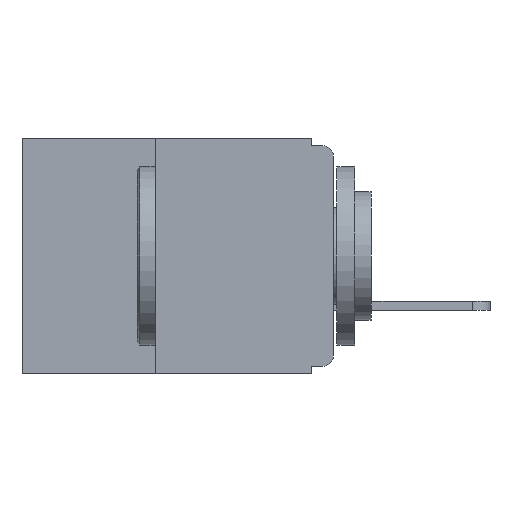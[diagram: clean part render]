
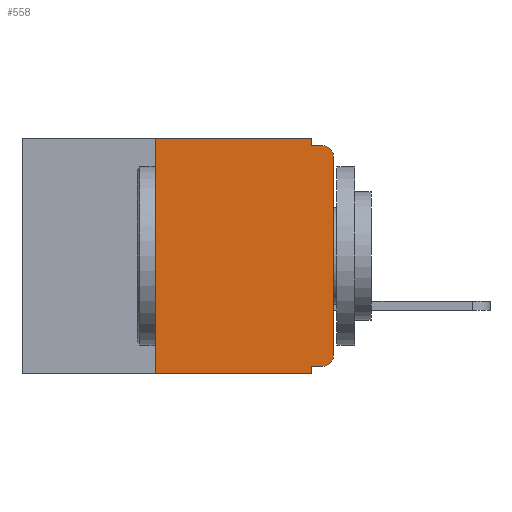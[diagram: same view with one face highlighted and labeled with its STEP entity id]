
A CAD part, left-side view. The second image highlights one B-rep face of the part: STEP entity #558.
In plain terms, the highlighted planar face has unit normal (-1, 0, 0).
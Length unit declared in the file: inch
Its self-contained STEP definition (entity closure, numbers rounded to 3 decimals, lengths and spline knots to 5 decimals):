
#59 = CARTESIAN_POINT ( 'NONE',  ( 0., 0.031, -0.01 ) ) ;
#419 = VERTEX_POINT ( 'NONE', #4689 ) ;
#448 = CARTESIAN_POINT ( 'NONE',  ( 0., 0.015, -0.025 ) ) ;
#558 = ADVANCED_FACE ( 'NONE', ( #9040 ), #2734, .F. ) ;
#847 = EDGE_LOOP ( 'NONE', ( #12731, #2607, #6334, #4284, #2708, #13436, #4653, #9390, #7043, #10764 ) ) ;
#981 = VERTEX_POINT ( 'NONE', #5485 ) ;
#991 = DIRECTION ( 'NONE',  ( 0., -1., 0. ) ) ;
#1083 = CIRCLE ( 'NONE', #13845, 0.015 ) ;
#1135 = CARTESIAN_POINT ( 'NONE',  ( 0., 0.031, -0.32 ) ) ;
#1449 = DIRECTION ( 'NONE',  ( -1., 0., 0. ) ) ;
#1473 = DIRECTION ( 'NONE',  ( 0., 1., 0. ) ) ;
#1557 = LINE ( 'NONE', #9419, #4744 ) ;
#1719 = VECTOR ( 'NONE', #3664, 39.37008 ) ;
#2457 = LINE ( 'NONE', #13601, #11210 ) ;
#2577 = EDGE_CURVE ( 'NONE', #981, #4015, #1083, .T. ) ;
#2607 = ORIENTED_EDGE ( 'NONE', *, *, #2577, .T. ) ;
#2708 = ORIENTED_EDGE ( 'NONE', *, *, #5765, .F. ) ;
#2734 = PLANE ( 'NONE',  #7742 ) ;
#2754 = DIRECTION ( 'NONE',  ( 0., 0., -1. ) ) ;
#3209 = EDGE_CURVE ( 'NONE', #8867, #8201, #5418, .T. ) ;
#3291 = CARTESIAN_POINT ( 'NONE',  ( 0., 0.25, -0.33 ) ) ;
#3367 = CARTESIAN_POINT ( 'NONE',  ( 0., 0., -0.305 ) ) ;
#3386 = EDGE_CURVE ( 'NONE', #4046, #8201, #7443, .T. ) ;
#3545 = VERTEX_POINT ( 'NONE', #59 ) ;
#3664 = DIRECTION ( 'NONE',  ( 0., 0., -1. ) ) ;
#4015 = VERTEX_POINT ( 'NONE', #8286 ) ;
#4018 = LINE ( 'NONE', #13266, #11631 ) ;
#4046 = VERTEX_POINT ( 'NONE', #11746 ) ;
#4284 = ORIENTED_EDGE ( 'NONE', *, *, #12924, .F. ) ;
#4653 = ORIENTED_EDGE ( 'NONE', *, *, #3386, .T. ) ;
#4667 = CARTESIAN_POINT ( 'NONE',  ( 0., 0.031, 0. ) ) ;
#4689 = CARTESIAN_POINT ( 'NONE',  ( 0., 0.015, -0.32 ) ) ;
#4744 = VECTOR ( 'NONE', #991, 39.37008 ) ;
#4830 = DIRECTION ( 'NONE',  ( 1., 0., 0. ) ) ;
#4857 = LINE ( 'NONE', #3291, #13137 ) ;
#5418 = LINE ( 'NONE', #11180, #1719 ) ;
#5485 = CARTESIAN_POINT ( 'NONE',  ( 0., 0., -0.025 ) ) ;
#5717 = CIRCLE ( 'NONE', #10807, 0.015 ) ;
#5765 = EDGE_CURVE ( 'NONE', #13213, #12849, #1557, .T. ) ;
#5987 = CARTESIAN_POINT ( 'NONE',  ( 0., 0.031, 0. ) ) ;
#6334 = ORIENTED_EDGE ( 'NONE', *, *, #9911, .F. ) ;
#7043 = ORIENTED_EDGE ( 'NONE', *, *, #13647, .F. ) ;
#7157 = CARTESIAN_POINT ( 'NONE',  ( 0., 0.25, 0. ) ) ;
#7209 = DIRECTION ( 'NONE',  ( 0., 0., -1. ) ) ;
#7434 = EDGE_CURVE ( 'NONE', #4046, #13213, #4857, .T. ) ;
#7443 = LINE ( 'NONE', #10498, #9984 ) ;
#7742 = AXIS2_PLACEMENT_3D ( 'NONE', #10250, #4830, #9224 ) ;
#7816 = EDGE_CURVE ( 'NONE', #419, #12351, #5717, .T. ) ;
#8201 = VERTEX_POINT ( 'NONE', #10678 ) ;
#8286 = CARTESIAN_POINT ( 'NONE',  ( 0., 0.015, -0.01 ) ) ;
#8867 = VERTEX_POINT ( 'NONE', #1135 ) ;
#8974 = DIRECTION ( 'NONE',  ( 0., 0., -1. ) ) ;
#9040 = FACE_OUTER_BOUND ( 'NONE', #847, .T. ) ;
#9224 = DIRECTION ( 'NONE',  ( 0., 0., -1. ) ) ;
#9390 = ORIENTED_EDGE ( 'NONE', *, *, #3209, .F. ) ;
#9419 = CARTESIAN_POINT ( 'NONE',  ( 0., 0.437, 0. ) ) ;
#9433 = DIRECTION ( 'NONE',  ( -1., 0., 0. ) ) ;
#9477 = CARTESIAN_POINT ( 'NONE',  ( 0., 0., 0. ) ) ;
#9524 = DIRECTION ( 'NONE',  ( 0., 0., 1. ) ) ;
#9848 = DIRECTION ( 'NONE',  ( 0., 0., 1. ) ) ;
#9911 = EDGE_CURVE ( 'NONE', #3545, #4015, #2457, .T. ) ;
#9984 = VECTOR ( 'NONE', #10549, 39.37008 ) ;
#10250 = CARTESIAN_POINT ( 'NONE',  ( 0., 0.437, 0. ) ) ;
#10278 = DIRECTION ( 'NONE',  ( 0., -1., 0. ) ) ;
#10498 = CARTESIAN_POINT ( 'NONE',  ( 0., 0.437, -0.33 ) ) ;
#10549 = DIRECTION ( 'NONE',  ( 0., -1., 0. ) ) ;
#10678 = CARTESIAN_POINT ( 'NONE',  ( 0., 0.031, -0.33 ) ) ;
#10764 = ORIENTED_EDGE ( 'NONE', *, *, #7816, .T. ) ;
#10807 = AXIS2_PLACEMENT_3D ( 'NONE', #13243, #1449, #8974 ) ;
#11180 = CARTESIAN_POINT ( 'NONE',  ( 0., 0.031, -0.33 ) ) ;
#11210 = VECTOR ( 'NONE', #10278, 39.37008 ) ;
#11463 = VECTOR ( 'NONE', #2754, 39.37008 ) ;
#11479 = LINE ( 'NONE', #9477, #13504 ) ;
#11627 = LINE ( 'NONE', #5987, #11463 ) ;
#11631 = VECTOR ( 'NONE', #1473, 39.37008 ) ;
#11746 = CARTESIAN_POINT ( 'NONE',  ( 0., 0.25, -0.33 ) ) ;
#12351 = VERTEX_POINT ( 'NONE', #3367 ) ;
#12731 = ORIENTED_EDGE ( 'NONE', *, *, #12756, .T. ) ;
#12756 = EDGE_CURVE ( 'NONE', #12351, #981, #11479, .T. ) ;
#12849 = VERTEX_POINT ( 'NONE', #4667 ) ;
#12924 = EDGE_CURVE ( 'NONE', #12849, #3545, #11627, .T. ) ;
#13137 = VECTOR ( 'NONE', #9848, 39.37008 ) ;
#13213 = VERTEX_POINT ( 'NONE', #7157 ) ;
#13243 = CARTESIAN_POINT ( 'NONE',  ( 0., 0.015, -0.305 ) ) ;
#13266 = CARTESIAN_POINT ( 'NONE',  ( 0., 0., -0.32 ) ) ;
#13436 = ORIENTED_EDGE ( 'NONE', *, *, #7434, .F. ) ;
#13504 = VECTOR ( 'NONE', #9524, 39.37008 ) ;
#13601 = CARTESIAN_POINT ( 'NONE',  ( 0., 0., -0.01 ) ) ;
#13647 = EDGE_CURVE ( 'NONE', #419, #8867, #4018, .T. ) ;
#13845 = AXIS2_PLACEMENT_3D ( 'NONE', #448, #9433, #7209 ) ;
